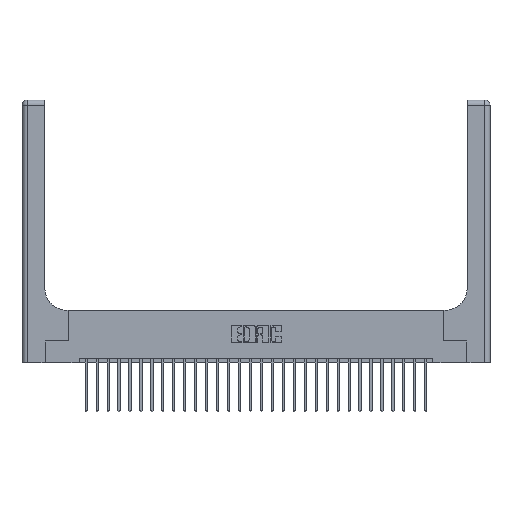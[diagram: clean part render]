
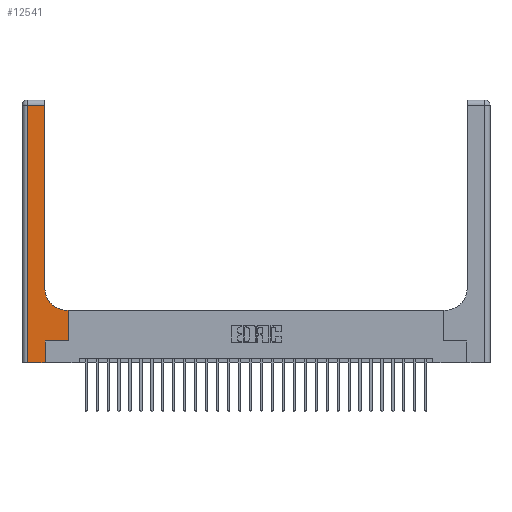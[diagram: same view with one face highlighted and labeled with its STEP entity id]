
A CAD part, top view. The second image highlights one B-rep face of the part: STEP entity #12541.
In plain terms, the highlighted planar face has unit normal (0, 0, 1).
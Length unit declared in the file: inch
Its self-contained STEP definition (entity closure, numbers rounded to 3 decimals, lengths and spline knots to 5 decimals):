
#657 = LINE ( 'NONE', #22147, #17211 ) ;
#1013 = CARTESIAN_POINT ( 'NONE',  ( 0.26, 3., 0.37 ) ) ;
#1104 = DIRECTION ( 'NONE',  ( 0., -1., 0. ) ) ;
#2138 = VECTOR ( 'NONE', #1104, 39.37008 ) ;
#2288 = VECTOR ( 'NONE', #17362, 39.37008 ) ;
#2640 = CARTESIAN_POINT ( 'NONE',  ( 0.51, 0.85, 0.37 ) ) ;
#2704 = LINE ( 'NONE', #24460, #24574 ) ;
#2740 = CARTESIAN_POINT ( 'NONE',  ( 0.265, 0.25, 0.37 ) ) ;
#3798 = EDGE_CURVE ( 'NONE', #9969, #25670, #12044, .T. ) ;
#4647 = AXIS2_PLACEMENT_3D ( 'NONE', #21575, #8932, #9295 ) ;
#4717 = ORIENTED_EDGE ( 'NONE', *, *, #14434, .T. ) ;
#4810 = PLANE ( 'NONE',  #4647 ) ;
#4834 = EDGE_CURVE ( 'NONE', #11212, #9969, #14272, .T. ) ;
#4893 = CARTESIAN_POINT ( 'NONE',  ( 0.26, 0.6, 0.37 ) ) ;
#5080 = LINE ( 'NONE', #12733, #9138 ) ;
#5143 = VECTOR ( 'NONE', #17972, 39.37008 ) ;
#5265 = EDGE_CURVE ( 'NONE', #18284, #22591, #657, .T. ) ;
#6082 = CARTESIAN_POINT ( 'NONE',  ( 0.528, 0.25, 0.37 ) ) ;
#7171 = CARTESIAN_POINT ( 'NONE',  ( 0., 2.94, 0.37 ) ) ;
#7413 = ORIENTED_EDGE ( 'NONE', *, *, #5265, .T. ) ;
#7477 = VECTOR ( 'NONE', #22520, 39.37008 ) ;
#7518 = LINE ( 'NONE', #9748, #7477 ) ;
#8930 = DIRECTION ( 'NONE',  ( -1., 0., 0. ) ) ;
#8932 = DIRECTION ( 'NONE',  ( 0., 0., -1. ) ) ;
#9137 = CARTESIAN_POINT ( 'NONE',  ( 0.265, 0., 0.37 ) ) ;
#9138 = VECTOR ( 'NONE', #25453, 39.37008 ) ;
#9295 = DIRECTION ( 'NONE',  ( -1., 0., 0. ) ) ;
#9332 = ORIENTED_EDGE ( 'NONE', *, *, #25847, .T. ) ;
#9748 = CARTESIAN_POINT ( 'NONE',  ( 0.528, 0.25, 0.37 ) ) ;
#9967 = DIRECTION ( 'NONE',  ( 1., 0., 0. ) ) ;
#9969 = VERTEX_POINT ( 'NONE', #25772 ) ;
#10000 = LINE ( 'NONE', #7171, #2288 ) ;
#11148 = EDGE_CURVE ( 'NONE', #12943, #18284, #2704, .T. ) ;
#11168 = ORIENTED_EDGE ( 'NONE', *, *, #25447, .T. ) ;
#11212 = VERTEX_POINT ( 'NONE', #22309 ) ;
#11305 = FACE_OUTER_BOUND ( 'NONE', #24410, .T. ) ;
#12044 = CIRCLE ( 'NONE', #16888, 0.25 ) ;
#12109 = EDGE_CURVE ( 'NONE', #17042, #27110, #10000, .T. ) ;
#12541 = ADVANCED_FACE ( 'NONE', ( #11305 ), #4810, .F. ) ;
#12733 = CARTESIAN_POINT ( 'NONE',  ( 0.265, 0.25, 0.37 ) ) ;
#12943 = VERTEX_POINT ( 'NONE', #25438 ) ;
#13344 = ORIENTED_EDGE ( 'NONE', *, *, #12109, .T. ) ;
#14272 = LINE ( 'NONE', #4893, #17243 ) ;
#14434 = EDGE_CURVE ( 'NONE', #25670, #17042, #21079, .T. ) ;
#14688 = EDGE_CURVE ( 'NONE', #21047, #11212, #7518, .T. ) ;
#14782 = CARTESIAN_POINT ( 'NONE',  ( 0.06, 2.94, 0.37 ) ) ;
#16888 = AXIS2_PLACEMENT_3D ( 'NONE', #2640, #25625, #21635 ) ;
#17042 = VERTEX_POINT ( 'NONE', #25439 ) ;
#17164 = ORIENTED_EDGE ( 'NONE', *, *, #4834, .T. ) ;
#17211 = VECTOR ( 'NONE', #24208, 39.37008 ) ;
#17243 = VECTOR ( 'NONE', #8930, 39.37008 ) ;
#17362 = DIRECTION ( 'NONE',  ( -1., 0., 0. ) ) ;
#17793 = CARTESIAN_POINT ( 'NONE',  ( 0.06, 3., 0.37 ) ) ;
#17972 = DIRECTION ( 'NONE',  ( 0., 1., 0. ) ) ;
#18284 = VERTEX_POINT ( 'NONE', #9137 ) ;
#18960 = ORIENTED_EDGE ( 'NONE', *, *, #3798, .T. ) ;
#20615 = CARTESIAN_POINT ( 'NONE',  ( 0.26, 0.85, 0.37 ) ) ;
#21047 = VERTEX_POINT ( 'NONE', #6082 ) ;
#21079 = LINE ( 'NONE', #1013, #5143 ) ;
#21575 = CARTESIAN_POINT ( 'NONE',  ( 0., 3., 0.37 ) ) ;
#21635 = DIRECTION ( 'NONE',  ( 1., 0., 0. ) ) ;
#21794 = ORIENTED_EDGE ( 'NONE', *, *, #14688, .T. ) ;
#22147 = CARTESIAN_POINT ( 'NONE',  ( 0.265, 0., 0.37 ) ) ;
#22309 = CARTESIAN_POINT ( 'NONE',  ( 0.528, 0.6, 0.37 ) ) ;
#22520 = DIRECTION ( 'NONE',  ( 0., 1., 0. ) ) ;
#22591 = VERTEX_POINT ( 'NONE', #2740 ) ;
#23528 = ORIENTED_EDGE ( 'NONE', *, *, #11148, .T. ) ;
#24208 = DIRECTION ( 'NONE',  ( 0., 1., 0. ) ) ;
#24410 = EDGE_LOOP ( 'NONE', ( #4717, #13344, #11168, #23528, #7413, #9332, #21794, #17164, #18960 ) ) ;
#24460 = CARTESIAN_POINT ( 'NONE',  ( 0., 0., 0.37 ) ) ;
#24574 = VECTOR ( 'NONE', #9967, 39.37008 ) ;
#24677 = LINE ( 'NONE', #17793, #2138 ) ;
#25438 = CARTESIAN_POINT ( 'NONE',  ( 0.06, 0., 0.37 ) ) ;
#25439 = CARTESIAN_POINT ( 'NONE',  ( 0.26, 2.94, 0.37 ) ) ;
#25447 = EDGE_CURVE ( 'NONE', #27110, #12943, #24677, .T. ) ;
#25453 = DIRECTION ( 'NONE',  ( 1., 0., 0. ) ) ;
#25625 = DIRECTION ( 'NONE',  ( 0., 0., -1. ) ) ;
#25670 = VERTEX_POINT ( 'NONE', #20615 ) ;
#25772 = CARTESIAN_POINT ( 'NONE',  ( 0.51, 0.6, 0.37 ) ) ;
#25847 = EDGE_CURVE ( 'NONE', #22591, #21047, #5080, .T. ) ;
#27110 = VERTEX_POINT ( 'NONE', #14782 ) ;
